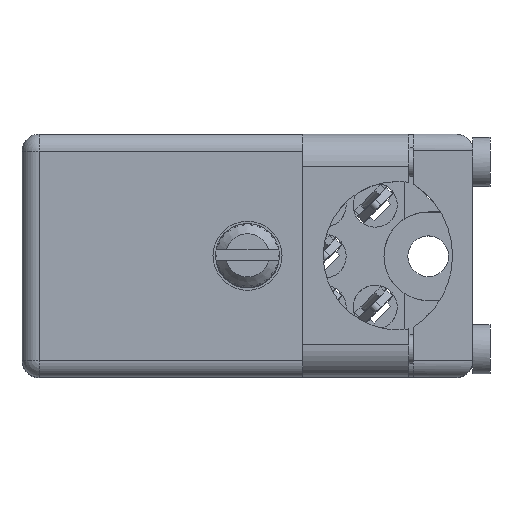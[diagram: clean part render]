
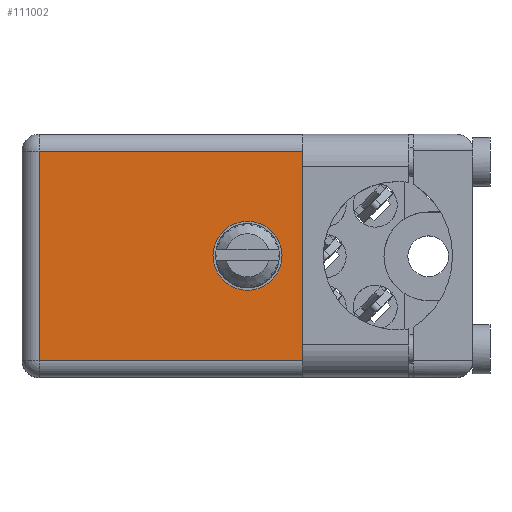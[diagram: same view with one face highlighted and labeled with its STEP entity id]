
A CAD part, top view. The second image highlights one B-rep face of the part: STEP entity #111002.
In plain terms, the highlighted face is planar.
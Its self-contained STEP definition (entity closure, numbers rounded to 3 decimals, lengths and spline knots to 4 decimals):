
#28 = DIRECTION ( 'NONE',  ( 1., 0., 0. ) ) ;
#3732 = VECTOR ( 'NONE', #59950, 39.3701 ) ;
#4489 = DIRECTION ( 'NONE',  ( 0., 0., 1. ) ) ;
#5230 = DIRECTION ( 'NONE',  ( 0., 0., 1. ) ) ;
#6978 = AXIS2_PLACEMENT_3D ( 'NONE', #161915, #47574, #4489 ) ;
#7027 = LINE ( 'NONE', #62321, #88012 ) ;
#9561 = VERTEX_POINT ( 'NONE', #28870 ) ;
#10439 = LINE ( 'NONE', #108800, #25415 ) ;
#10696 = CARTESIAN_POINT ( 'NONE',  ( 0.6625, 0.906, -0.256 ) ) ;
#12793 = ORIENTED_EDGE ( 'NONE', *, *, #58030, .T. ) ;
#15520 = EDGE_CURVE ( 'NONE', #159559, #156324, #128400, .T. ) ;
#17250 = ORIENTED_EDGE ( 'NONE', *, *, #174888, .T. ) ;
#17251 = CARTESIAN_POINT ( 'NONE',  ( 1.15, 0.906, -0.665 ) ) ;
#18100 = CARTESIAN_POINT ( 'NONE',  ( 0.865, 0.906, -0.1125 ) ) ;
#18308 = DIRECTION ( 'NONE',  ( 1., 0., 0. ) ) ;
#25415 = VECTOR ( 'NONE', #166929, 39.3701 ) ;
#28870 = CARTESIAN_POINT ( 'NONE',  ( 0.6625, 0.906, -0.459 ) ) ;
#31970 = ORIENTED_EDGE ( 'NONE', *, *, #87156, .T. ) ;
#33365 = DIRECTION ( 'NONE',  ( 0., 0., 1. ) ) ;
#33816 = CARTESIAN_POINT ( 'NONE',  ( 0.865, 0.906, -0.6025 ) ) ;
#36267 = EDGE_CURVE ( 'NONE', #110723, #156324, #56176, .T. ) ;
#37223 = VECTOR ( 'NONE', #140511, 39.3701 ) ;
#42836 = FACE_OUTER_BOUND ( 'NONE', #181509, .T. ) ;
#43094 = VECTOR ( 'NONE', #5230, 39.3701 ) ;
#43761 = PLANE ( 'NONE',  #96250 ) ;
#47574 = DIRECTION ( 'NONE',  ( 0., 1., 0. ) ) ;
#49363 = VECTOR ( 'NONE', #28, 39.3701 ) ;
#53774 = ORIENTED_EDGE ( 'NONE', *, *, #153286, .T. ) ;
#56176 = LINE ( 'NONE', #154628, #37223 ) ;
#58030 = EDGE_CURVE ( 'NONE', #89841, #150917, #118042, .T. ) ;
#58729 = DIRECTION ( 'NONE',  ( 0., 1., 0. ) ) ;
#59950 = DIRECTION ( 'NONE',  ( 0., 0., -1. ) ) ;
#60277 = DIRECTION ( 'NONE',  ( -1., 0., 0. ) ) ;
#62321 = CARTESIAN_POINT ( 'NONE',  ( 0.865, 0.906, -0.6025 ) ) ;
#63332 = VECTOR ( 'NONE', #60277, 39.3701 ) ;
#66289 = CARTESIAN_POINT ( 'NONE',  ( 0., 0.906, -0.665 ) ) ;
#69261 = CARTESIAN_POINT ( 'NONE',  ( 1.15, 0.906, -0.6025 ) ) ;
#69868 = CIRCLE ( 'NONE', #6978, 0.1015 ) ;
#70026 = LINE ( 'NONE', #66289, #168906 ) ;
#70859 = ORIENTED_EDGE ( 'NONE', *, *, #15520, .T. ) ;
#73732 = CARTESIAN_POINT ( 'NONE',  ( 0., 0.906, -0.715 ) ) ;
#81293 = AXIS2_PLACEMENT_3D ( 'NONE', #168033, #153051, #112696 ) ;
#87156 = EDGE_CURVE ( 'NONE', #109880, #159559, #131726, .T. ) ;
#88012 = VECTOR ( 'NONE', #18308, 39.3701 ) ;
#89656 = ORIENTED_EDGE ( 'NONE', *, *, #178603, .F. ) ;
#89807 = ORIENTED_EDGE ( 'NONE', *, *, #112393, .F. ) ;
#89841 = VERTEX_POINT ( 'NONE', #119562 ) ;
#93772 = ORIENTED_EDGE ( 'NONE', *, *, #160157, .F. ) ;
#96250 = AXIS2_PLACEMENT_3D ( 'NONE', #73732, #58729, #33365 ) ;
#102723 = ORIENTED_EDGE ( 'NONE', *, *, #129131, .T. ) ;
#108800 = CARTESIAN_POINT ( 'NONE',  ( 1.15, 0.906, -0.715 ) ) ;
#109880 = VERTEX_POINT ( 'NONE', #163388 ) ;
#110723 = VERTEX_POINT ( 'NONE', #161518 ) ;
#111002 = ADVANCED_FACE ( 'NONE', ( #42836, #167534 ), #43761, .T. ) ;
#112393 = EDGE_CURVE ( 'NONE', #9561, #125330, #183110, .T. ) ;
#112696 = DIRECTION ( 'NONE',  ( 0., 0., 1. ) ) ;
#118042 = LINE ( 'NONE', #130254, #3732 ) ;
#119426 = CARTESIAN_POINT ( 'NONE',  ( 0.05, 0.906, -0.05 ) ) ;
#119562 = CARTESIAN_POINT ( 'NONE',  ( 0.865, 0.906, -0.1125 ) ) ;
#125330 = VERTEX_POINT ( 'NONE', #10696 ) ;
#128400 = LINE ( 'NONE', #144325, #49363 ) ;
#129131 = EDGE_CURVE ( 'NONE', #110723, #89841, #158720, .T. ) ;
#130254 = CARTESIAN_POINT ( 'NONE',  ( 0.865, 0.906, -0.1125 ) ) ;
#131726 = LINE ( 'NONE', #176745, #43094 ) ;
#140511 = DIRECTION ( 'NONE',  ( 0., 0., 1. ) ) ;
#144325 = CARTESIAN_POINT ( 'NONE',  ( 1.15, 0.906, -0.05 ) ) ;
#150473 = EDGE_LOOP ( 'NONE', ( #93772, #89807 ) ) ;
#150917 = VERTEX_POINT ( 'NONE', #33816 ) ;
#151130 = ORIENTED_EDGE ( 'NONE', *, *, #36267, .F. ) ;
#153051 = DIRECTION ( 'NONE',  ( 0., 1., 0. ) ) ;
#153286 = EDGE_CURVE ( 'NONE', #180515, #109880, #70026, .T. ) ;
#153464 = DIRECTION ( 'NONE',  ( -1., 0., 0. ) ) ;
#154628 = CARTESIAN_POINT ( 'NONE',  ( 1.15, 0.906, -0.715 ) ) ;
#156324 = VERTEX_POINT ( 'NONE', #169867 ) ;
#158720 = LINE ( 'NONE', #18100, #63332 ) ;
#159559 = VERTEX_POINT ( 'NONE', #119426 ) ;
#160157 = EDGE_CURVE ( 'NONE', #125330, #9561, #69868, .T. ) ;
#161086 = VERTEX_POINT ( 'NONE', #69261 ) ;
#161518 = CARTESIAN_POINT ( 'NONE',  ( 1.15, 0.906, -0.1125 ) ) ;
#161915 = CARTESIAN_POINT ( 'NONE',  ( 0.6625, 0.906, -0.3575 ) ) ;
#163388 = CARTESIAN_POINT ( 'NONE',  ( 0.05, 0.906, -0.665 ) ) ;
#166929 = DIRECTION ( 'NONE',  ( 0., 0., 1. ) ) ;
#167534 = FACE_BOUND ( 'NONE', #150473, .T. ) ;
#168033 = CARTESIAN_POINT ( 'NONE',  ( 0.6625, 0.906, -0.3575 ) ) ;
#168906 = VECTOR ( 'NONE', #153464, 39.3701 ) ;
#169867 = CARTESIAN_POINT ( 'NONE',  ( 1.15, 0.906, -0.05 ) ) ;
#174888 = EDGE_CURVE ( 'NONE', #150917, #161086, #7027, .T. ) ;
#176745 = CARTESIAN_POINT ( 'NONE',  ( 0.05, 0.906, -0.715 ) ) ;
#178603 = EDGE_CURVE ( 'NONE', #180515, #161086, #10439, .T. ) ;
#180515 = VERTEX_POINT ( 'NONE', #17251 ) ;
#181509 = EDGE_LOOP ( 'NONE', ( #31970, #70859, #151130, #102723, #12793, #17250, #89656, #53774 ) ) ;
#183110 = CIRCLE ( 'NONE', #81293, 0.1015 ) ;
